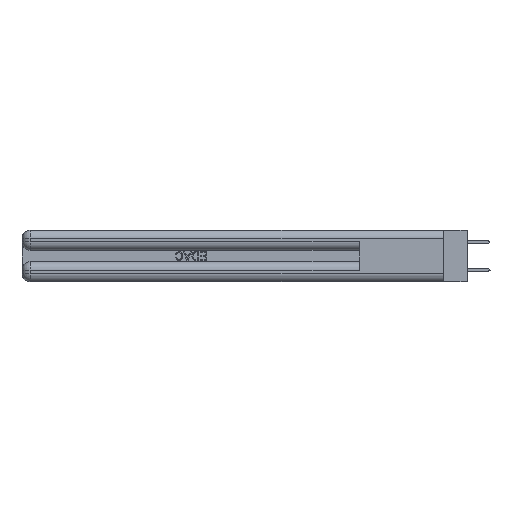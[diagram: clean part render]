
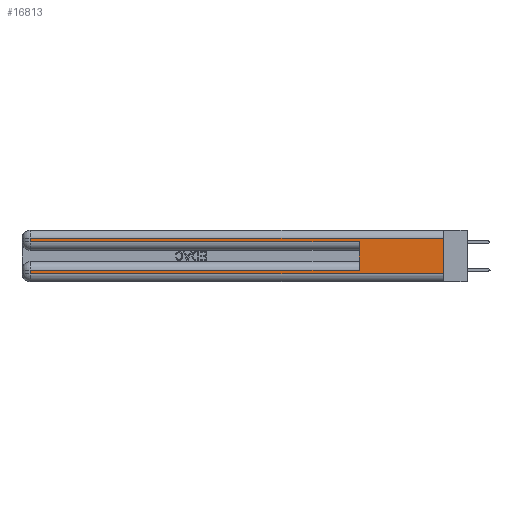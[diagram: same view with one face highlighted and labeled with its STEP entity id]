
A CAD part, left-side view. The second image highlights one B-rep face of the part: STEP entity #16813.
In plain terms, the highlighted planar face has unit normal (-1, 0, 0).
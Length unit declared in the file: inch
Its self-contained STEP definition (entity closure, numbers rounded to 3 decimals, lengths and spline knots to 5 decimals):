
#1262 = DIRECTION ( 'NONE',  ( 0., 0., -1. ) ) ;
#1775 = CARTESIAN_POINT ( 'NONE',  ( 0., 0., 0.37 ) ) ;
#2616 = VECTOR ( 'NONE', #1262, 39.37008 ) ;
#4682 = VECTOR ( 'NONE', #35788, 39.37008 ) ;
#4693 = ORIENTED_EDGE ( 'NONE', *, *, #8663, .T. ) ;
#5561 = VERTEX_POINT ( 'NONE', #21846 ) ;
#5572 = CARTESIAN_POINT ( 'NONE',  ( 0., 2.94, 0.285 ) ) ;
#5770 = LINE ( 'NONE', #30153, #40475 ) ;
#6153 = VECTOR ( 'NONE', #18951, 39.37008 ) ;
#6365 = LINE ( 'NONE', #21511, #4682 ) ;
#6701 = VERTEX_POINT ( 'NONE', #22462 ) ;
#7970 = LINE ( 'NONE', #34421, #43227 ) ;
#8663 = EDGE_CURVE ( 'NONE', #27757, #26251, #24676, .T. ) ;
#8672 = EDGE_CURVE ( 'NONE', #12005, #27757, #30231, .T. ) ;
#10554 = VERTEX_POINT ( 'NONE', #5572 ) ;
#10746 = VERTEX_POINT ( 'NONE', #17002 ) ;
#11740 = ORIENTED_EDGE ( 'NONE', *, *, #12669, .T. ) ;
#12005 = VERTEX_POINT ( 'NONE', #26920 ) ;
#12205 = CARTESIAN_POINT ( 'NONE',  ( 0., 0., 0.31 ) ) ;
#12669 = EDGE_CURVE ( 'NONE', #5561, #6701, #36907, .T. ) ;
#13128 = LINE ( 'NONE', #36350, #39456 ) ;
#15878 = ORIENTED_EDGE ( 'NONE', *, *, #26835, .T. ) ;
#16390 = ORIENTED_EDGE ( 'NONE', *, *, #18547, .T. ) ;
#16636 = EDGE_CURVE ( 'NONE', #21480, #10746, #6365, .T. ) ;
#16813 = ADVANCED_FACE ( 'NONE', ( #43212 ), #25154, .F. ) ;
#16911 = ORIENTED_EDGE ( 'NONE', *, *, #8672, .T. ) ;
#17002 = CARTESIAN_POINT ( 'NONE',  ( 0., 0.6, 0.285 ) ) ;
#18547 = EDGE_CURVE ( 'NONE', #10554, #10746, #5770, .T. ) ;
#18951 = DIRECTION ( 'NONE',  ( 0., 1., 0. ) ) ;
#19491 = DIRECTION ( 'NONE',  ( 0., 1., 0. ) ) ;
#21480 = VERTEX_POINT ( 'NONE', #27126 ) ;
#21511 = CARTESIAN_POINT ( 'NONE',  ( 0., 0.6, 0.145 ) ) ;
#21846 = CARTESIAN_POINT ( 'NONE',  ( 0., 0., 0.31 ) ) ;
#22462 = CARTESIAN_POINT ( 'NONE',  ( 0., 2.94, 0.31 ) ) ;
#22749 = ORIENTED_EDGE ( 'NONE', *, *, #42542, .T. ) ;
#23071 = DIRECTION ( 'NONE',  ( 0., 0., -1. ) ) ;
#24676 = LINE ( 'NONE', #25795, #31804 ) ;
#24875 = DIRECTION ( 'NONE',  ( 0., 0., -1. ) ) ;
#24894 = CARTESIAN_POINT ( 'NONE',  ( 0., 2.94, 0.06 ) ) ;
#25154 = PLANE ( 'NONE',  #38280 ) ;
#25795 = CARTESIAN_POINT ( 'NONE',  ( 0., 0., 0.06 ) ) ;
#26183 = ORIENTED_EDGE ( 'NONE', *, *, #35330, .F. ) ;
#26251 = VERTEX_POINT ( 'NONE', #30424 ) ;
#26450 = DIRECTION ( 'NONE',  ( 0., -1., 0. ) ) ;
#26835 = EDGE_CURVE ( 'NONE', #21480, #12005, #13128, .T. ) ;
#26920 = CARTESIAN_POINT ( 'NONE',  ( 0., 2.94, 0.085 ) ) ;
#27126 = CARTESIAN_POINT ( 'NONE',  ( 0., 0.6, 0.085 ) ) ;
#27757 = VERTEX_POINT ( 'NONE', #24894 ) ;
#30153 = CARTESIAN_POINT ( 'NONE',  ( 0., 0., 0.285 ) ) ;
#30231 = LINE ( 'NONE', #44464, #42349 ) ;
#30424 = CARTESIAN_POINT ( 'NONE',  ( 0., 0., 0.06 ) ) ;
#30641 = LINE ( 'NONE', #42812, #2616 ) ;
#31476 = DIRECTION ( 'NONE',  ( 0., 0., -1. ) ) ;
#31804 = VECTOR ( 'NONE', #32847, 39.37008 ) ;
#32847 = DIRECTION ( 'NONE',  ( 0., -1., 0. ) ) ;
#34421 = CARTESIAN_POINT ( 'NONE',  ( 0., 2.94, 0.37 ) ) ;
#35249 = ORIENTED_EDGE ( 'NONE', *, *, #16636, .F. ) ;
#35330 = EDGE_CURVE ( 'NONE', #5561, #26251, #30641, .T. ) ;
#35788 = DIRECTION ( 'NONE',  ( 0., 0., 1. ) ) ;
#36350 = CARTESIAN_POINT ( 'NONE',  ( 0., 0., 0.085 ) ) ;
#36907 = LINE ( 'NONE', #12205, #6153 ) ;
#37111 = DIRECTION ( 'NONE',  ( 1., 0., 0. ) ) ;
#38280 = AXIS2_PLACEMENT_3D ( 'NONE', #1775, #37111, #24875 ) ;
#39456 = VECTOR ( 'NONE', #19491, 39.37008 ) ;
#40475 = VECTOR ( 'NONE', #26450, 39.37008 ) ;
#42349 = VECTOR ( 'NONE', #23071, 39.37008 ) ;
#42542 = EDGE_CURVE ( 'NONE', #6701, #10554, #7970, .T. ) ;
#42812 = CARTESIAN_POINT ( 'NONE',  ( 0., 0., 0.37 ) ) ;
#43212 = FACE_OUTER_BOUND ( 'NONE', #44419, .T. ) ;
#43227 = VECTOR ( 'NONE', #31476, 39.37008 ) ;
#44419 = EDGE_LOOP ( 'NONE', ( #26183, #11740, #22749, #16390, #35249, #15878, #16911, #4693 ) ) ;
#44464 = CARTESIAN_POINT ( 'NONE',  ( 0., 2.94, 0.37 ) ) ;
